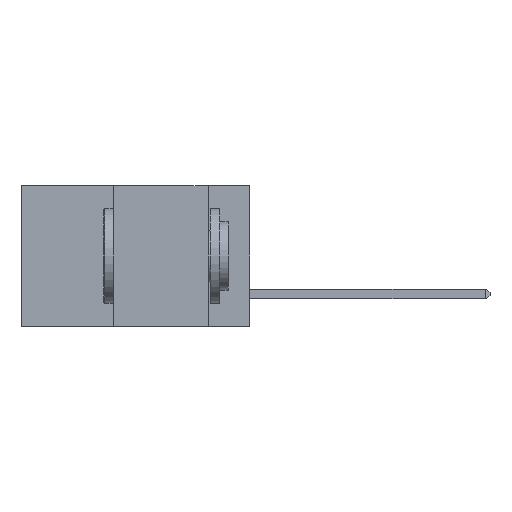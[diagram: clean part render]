
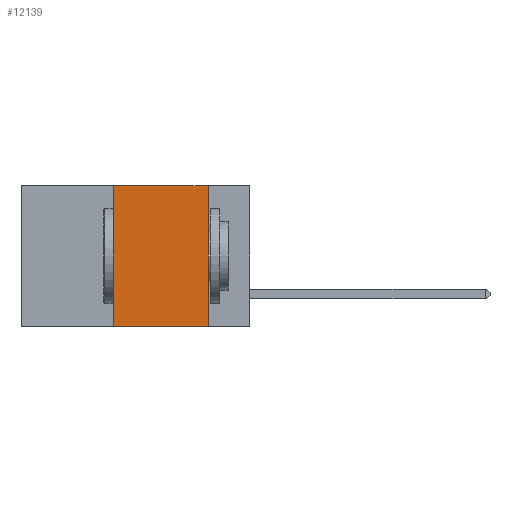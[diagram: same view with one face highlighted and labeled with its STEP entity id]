
A CAD part, left-side view. The second image highlights one B-rep face of the part: STEP entity #12139.
In plain terms, the highlighted planar face has unit normal (-1, 0, 0).
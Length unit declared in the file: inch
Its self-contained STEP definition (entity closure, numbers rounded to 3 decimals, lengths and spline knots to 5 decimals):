
#1154 = LINE ( 'NONE', #12125, #5886 ) ;
#1825 = CARTESIAN_POINT ( 'NONE',  ( 0., 0.6, -0.37 ) ) ;
#2548 = CARTESIAN_POINT ( 'NONE',  ( 0., 0.36, 0. ) ) ;
#2629 = VERTEX_POINT ( 'NONE', #3651 ) ;
#2779 = LINE ( 'NONE', #11339, #22536 ) ;
#3284 = DIRECTION ( 'NONE',  ( 0., 0., -1. ) ) ;
#3545 = VECTOR ( 'NONE', #14898, 39.37008 ) ;
#3651 = CARTESIAN_POINT ( 'NONE',  ( 0., 0.11, 0. ) ) ;
#4149 = ORIENTED_EDGE ( 'NONE', *, *, #19534, .F. ) ;
#5886 = VECTOR ( 'NONE', #10127, 39.37008 ) ;
#6533 = EDGE_LOOP ( 'NONE', ( #18102, #13541, #4149, #9520 ) ) ;
#7793 = VECTOR ( 'NONE', #13841, 39.37008 ) ;
#8722 = EDGE_CURVE ( 'NONE', #15297, #18273, #13107, .T. ) ;
#8796 = EDGE_CURVE ( 'NONE', #12992, #2629, #1154, .T. ) ;
#9520 = ORIENTED_EDGE ( 'NONE', *, *, #8722, .T. ) ;
#10127 = DIRECTION ( 'NONE',  ( 0., -1., 0. ) ) ;
#11339 = CARTESIAN_POINT ( 'NONE',  ( 0., 0.11, 0. ) ) ;
#11994 = DIRECTION ( 'NONE',  ( 1., 0., 0. ) ) ;
#12125 = CARTESIAN_POINT ( 'NONE',  ( 0., 0.6, 0. ) ) ;
#12139 = ADVANCED_FACE ( 'NONE', ( #14494 ), #25484, .F. ) ;
#12992 = VERTEX_POINT ( 'NONE', #2548 ) ;
#13107 = LINE ( 'NONE', #1825, #7793 ) ;
#13541 = ORIENTED_EDGE ( 'NONE', *, *, #8796, .F. ) ;
#13841 = DIRECTION ( 'NONE',  ( 0., -1., 0. ) ) ;
#14494 = FACE_OUTER_BOUND ( 'NONE', #6533, .T. ) ;
#14705 = CARTESIAN_POINT ( 'NONE',  ( 0., 0.11, -0.37 ) ) ;
#14898 = DIRECTION ( 'NONE',  ( 0., 0., 1. ) ) ;
#15297 = VERTEX_POINT ( 'NONE', #18976 ) ;
#15337 = EDGE_CURVE ( 'NONE', #2629, #18273, #2779, .T. ) ;
#17306 = AXIS2_PLACEMENT_3D ( 'NONE', #23625, #11994, #25572 ) ;
#18102 = ORIENTED_EDGE ( 'NONE', *, *, #15337, .F. ) ;
#18273 = VERTEX_POINT ( 'NONE', #14705 ) ;
#18976 = CARTESIAN_POINT ( 'NONE',  ( 0., 0.36, -0.37 ) ) ;
#19534 = EDGE_CURVE ( 'NONE', #15297, #12992, #24542, .T. ) ;
#22536 = VECTOR ( 'NONE', #3284, 39.37008 ) ;
#23625 = CARTESIAN_POINT ( 'NONE',  ( 0., 0.6, 0. ) ) ;
#24542 = LINE ( 'NONE', #24565, #3545 ) ;
#24565 = CARTESIAN_POINT ( 'NONE',  ( 0., 0.36, 0. ) ) ;
#25484 = PLANE ( 'NONE',  #17306 ) ;
#25572 = DIRECTION ( 'NONE',  ( 0., 0., -1. ) ) ;
